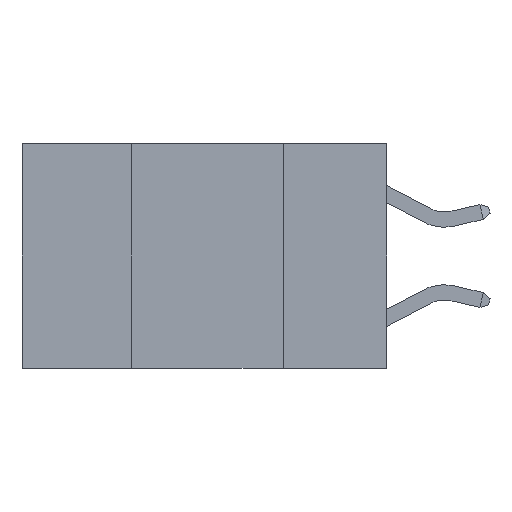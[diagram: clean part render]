
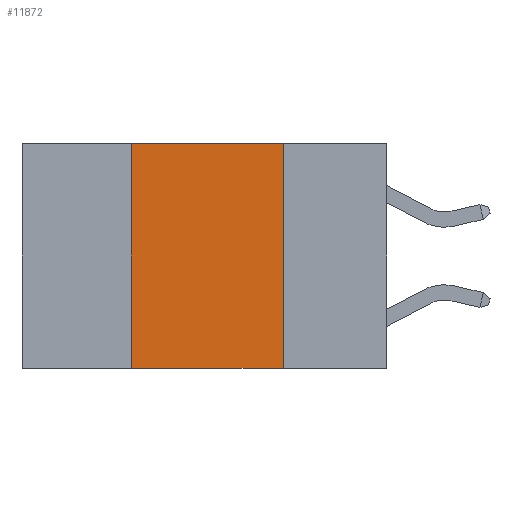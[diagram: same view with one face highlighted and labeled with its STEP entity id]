
A CAD part, left-side view. The second image highlights one B-rep face of the part: STEP entity #11872.
In plain terms, the highlighted planar face has unit normal (-1, 0, 0).
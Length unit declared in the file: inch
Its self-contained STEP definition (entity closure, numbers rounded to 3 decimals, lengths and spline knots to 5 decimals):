
#875 = CARTESIAN_POINT ( 'NONE',  ( 0., 0.6, 0. ) ) ;
#2924 = DIRECTION ( 'NONE',  ( 0., 0., -1. ) ) ;
#4039 = LINE ( 'NONE', #15921, #14617 ) ;
#4391 = ORIENTED_EDGE ( 'NONE', *, *, #24265, .F. ) ;
#5304 = CARTESIAN_POINT ( 'NONE',  ( 0., 0.17, 0. ) ) ;
#5564 = CARTESIAN_POINT ( 'NONE',  ( 0., 0.17, 0. ) ) ;
#5591 = VECTOR ( 'NONE', #21996, 39.37008 ) ;
#6118 = VECTOR ( 'NONE', #2924, 39.37008 ) ;
#6584 = DIRECTION ( 'NONE',  ( 1., 0., 0. ) ) ;
#6941 = LINE ( 'NONE', #5304, #6118 ) ;
#9967 = VERTEX_POINT ( 'NONE', #16729 ) ;
#10401 = EDGE_CURVE ( 'NONE', #21384, #20552, #6941, .T. ) ;
#10748 = LINE ( 'NONE', #18346, #24524 ) ;
#11872 = ADVANCED_FACE ( 'NONE', ( #22294 ), #23916, .F. ) ;
#11963 = ORIENTED_EDGE ( 'NONE', *, *, #10401, .F. ) ;
#13181 = VERTEX_POINT ( 'NONE', #14845 ) ;
#14463 = DIRECTION ( 'NONE',  ( 0., 0., -1. ) ) ;
#14617 = VECTOR ( 'NONE', #19416, 39.37008 ) ;
#14845 = CARTESIAN_POINT ( 'NONE',  ( 0., 0.42, -0.37 ) ) ;
#15301 = EDGE_CURVE ( 'NONE', #13181, #20552, #4039, .T. ) ;
#15921 = CARTESIAN_POINT ( 'NONE',  ( 0., 0.6, -0.37 ) ) ;
#16269 = LINE ( 'NONE', #24226, #5591 ) ;
#16729 = CARTESIAN_POINT ( 'NONE',  ( 0., 0.42, 0. ) ) ;
#16947 = EDGE_LOOP ( 'NONE', ( #11963, #19301, #4391, #22846 ) ) ;
#17990 = CARTESIAN_POINT ( 'NONE',  ( 0., 0.17, -0.37 ) ) ;
#18346 = CARTESIAN_POINT ( 'NONE',  ( 0., 0.6, 0. ) ) ;
#19301 = ORIENTED_EDGE ( 'NONE', *, *, #19375, .F. ) ;
#19375 = EDGE_CURVE ( 'NONE', #9967, #21384, #10748, .T. ) ;
#19416 = DIRECTION ( 'NONE',  ( 0., -1., 0. ) ) ;
#20552 = VERTEX_POINT ( 'NONE', #17990 ) ;
#21384 = VERTEX_POINT ( 'NONE', #5564 ) ;
#21996 = DIRECTION ( 'NONE',  ( 0., 0., 1. ) ) ;
#22294 = FACE_OUTER_BOUND ( 'NONE', #16947, .T. ) ;
#22520 = AXIS2_PLACEMENT_3D ( 'NONE', #875, #6584, #14463 ) ;
#22846 = ORIENTED_EDGE ( 'NONE', *, *, #15301, .T. ) ;
#23916 = PLANE ( 'NONE',  #22520 ) ;
#24203 = DIRECTION ( 'NONE',  ( 0., -1., 0. ) ) ;
#24226 = CARTESIAN_POINT ( 'NONE',  ( 0., 0.42, 0. ) ) ;
#24265 = EDGE_CURVE ( 'NONE', #13181, #9967, #16269, .T. ) ;
#24524 = VECTOR ( 'NONE', #24203, 39.37008 ) ;
